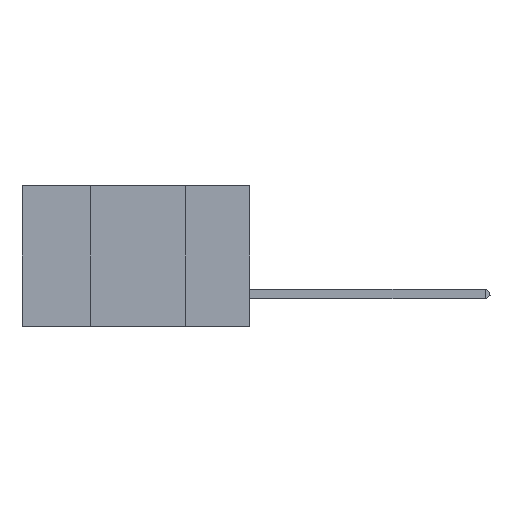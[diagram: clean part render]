
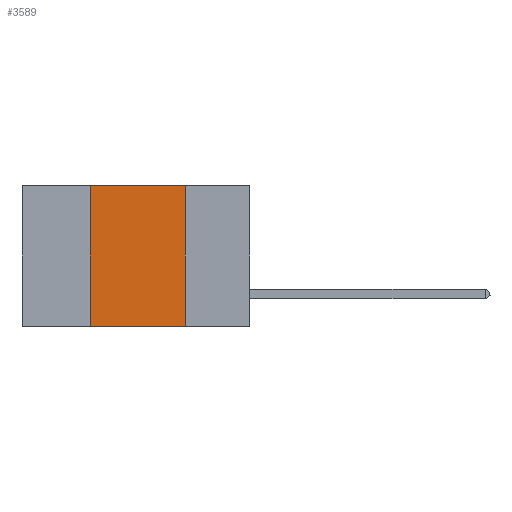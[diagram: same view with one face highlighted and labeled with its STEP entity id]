
A CAD part, left-side view. The second image highlights one B-rep face of the part: STEP entity #3589.
In plain terms, the highlighted planar face has unit normal (-1, 0, 0).
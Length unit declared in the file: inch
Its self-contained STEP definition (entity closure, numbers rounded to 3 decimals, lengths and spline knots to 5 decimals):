
#263 = CARTESIAN_POINT ( 'NONE',  ( 0., 0.6, 0. ) ) ;
#1001 = ORIENTED_EDGE ( 'NONE', *, *, #12590, .F. ) ;
#1047 = CARTESIAN_POINT ( 'NONE',  ( 0., 0.17, 0. ) ) ;
#1196 = EDGE_CURVE ( 'NONE', #7805, #15611, #6387, .T. ) ;
#2975 = CARTESIAN_POINT ( 'NONE',  ( 0., 0.17, -0.37 ) ) ;
#3456 = VERTEX_POINT ( 'NONE', #2975 ) ;
#3589 = ADVANCED_FACE ( 'NONE', ( #7006 ), #4403, .F. ) ;
#3988 = VERTEX_POINT ( 'NONE', #17671 ) ;
#4305 = VECTOR ( 'NONE', #8246, 39.37008 ) ;
#4403 = PLANE ( 'NONE',  #10373 ) ;
#4705 = CARTESIAN_POINT ( 'NONE',  ( 0., 0.42, 0. ) ) ;
#5004 = EDGE_LOOP ( 'NONE', ( #7096, #1001, #16221, #13844 ) ) ;
#5589 = CARTESIAN_POINT ( 'NONE',  ( 0., 0.42, 0. ) ) ;
#5770 = CARTESIAN_POINT ( 'NONE',  ( 0., 0.6, 0. ) ) ;
#5996 = DIRECTION ( 'NONE',  ( 1., 0., 0. ) ) ;
#6198 = EDGE_CURVE ( 'NONE', #3988, #3456, #8234, .T. ) ;
#6235 = DIRECTION ( 'NONE',  ( 0., 0., 1. ) ) ;
#6387 = LINE ( 'NONE', #4705, #12719 ) ;
#7006 = FACE_OUTER_BOUND ( 'NONE', #5004, .T. ) ;
#7066 = CARTESIAN_POINT ( 'NONE',  ( 0., 0.6, -0.37 ) ) ;
#7096 = ORIENTED_EDGE ( 'NONE', *, *, #6198, .F. ) ;
#7805 = VERTEX_POINT ( 'NONE', #14794 ) ;
#8234 = LINE ( 'NONE', #1047, #17172 ) ;
#8246 = DIRECTION ( 'NONE',  ( 0., -1., 0. ) ) ;
#8617 = DIRECTION ( 'NONE',  ( 0., -1., 0. ) ) ;
#9336 = LINE ( 'NONE', #5770, #12793 ) ;
#10373 = AXIS2_PLACEMENT_3D ( 'NONE', #263, #5996, #13269 ) ;
#10912 = DIRECTION ( 'NONE',  ( 0., 0., -1. ) ) ;
#11615 = EDGE_CURVE ( 'NONE', #7805, #3456, #17434, .T. ) ;
#12590 = EDGE_CURVE ( 'NONE', #15611, #3988, #9336, .T. ) ;
#12719 = VECTOR ( 'NONE', #6235, 39.37008 ) ;
#12793 = VECTOR ( 'NONE', #8617, 39.37008 ) ;
#13269 = DIRECTION ( 'NONE',  ( 0., 0., -1. ) ) ;
#13844 = ORIENTED_EDGE ( 'NONE', *, *, #11615, .T. ) ;
#14794 = CARTESIAN_POINT ( 'NONE',  ( 0., 0.42, -0.37 ) ) ;
#15611 = VERTEX_POINT ( 'NONE', #5589 ) ;
#16221 = ORIENTED_EDGE ( 'NONE', *, *, #1196, .F. ) ;
#17172 = VECTOR ( 'NONE', #10912, 39.37008 ) ;
#17434 = LINE ( 'NONE', #7066, #4305 ) ;
#17671 = CARTESIAN_POINT ( 'NONE',  ( 0., 0.17, 0. ) ) ;
